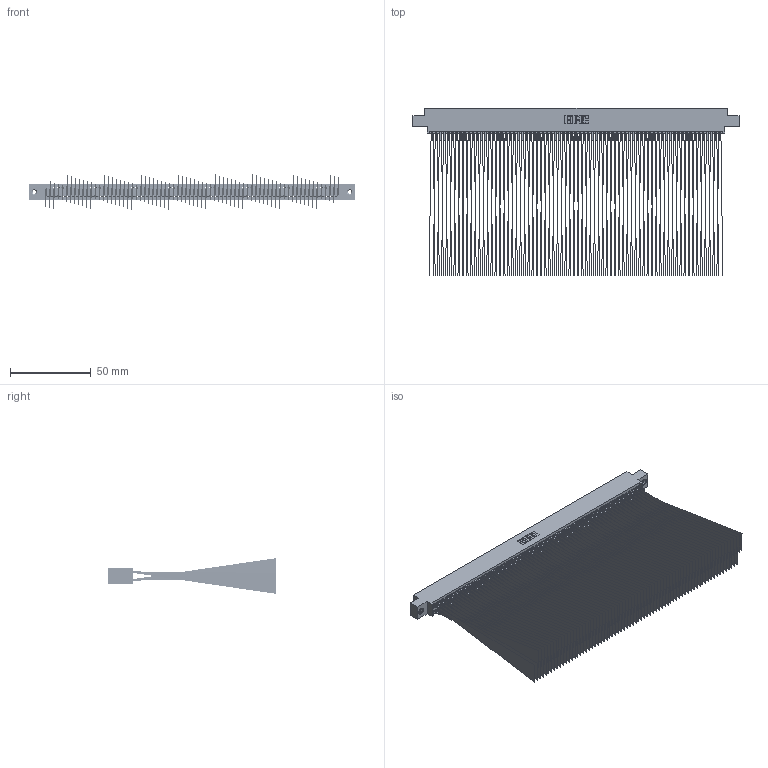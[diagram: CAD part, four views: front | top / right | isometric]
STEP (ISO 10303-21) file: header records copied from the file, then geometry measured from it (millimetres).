
FILE_DESCRIPTION (( 'STEP AP203' ), '1' );
FILE_NAME ('345-142-520-808.STEP', '2018-10-21T03:31:19', ( '' ), ( '' ), 'SwSTEP 2.0', 'SolidWorks 2016', '' );
FILE_SCHEMA (( 'CONFIG_CONTROL_DESIGN' ));
Length unit declared in the file: inch
Products named in the file (4): 345-292-001_345-293-120; 345-250-001_345-250-003-102; 345-142-520-808; 345 Part_0.170 Offset - 0.156 Dia-TI
Assembly tree (145 placements, depth 2):
  345-142-520-808
    345 Part_0.170 Offset - 0.156 Dia-TI
    345-292-001_345-293-120  x142
    345-250-001_345-250-003-102  x2
Bounding box: 201.55 x 103.28 x 22 mm (x, y, z)
Volume: 58210.1 mm3; surface area: 214268.8 mm2
Topology: 145 solids, 145 shells, 7858 faces, 22783 edges, 14944 vertices
Faces by surface type: plane 5086, cylinder 2756, cone 12, torus 4
Entity records: 53236 total; most frequent: CARTESIAN_POINT 8891, ORIENTED_EDGE 8806, DIRECTION 7817, EDGE_CURVE 4403, LINE 3963, VECTOR 3963, VERTEX_POINT 2928, AXIS2_PLACEMENT_3D 1927
